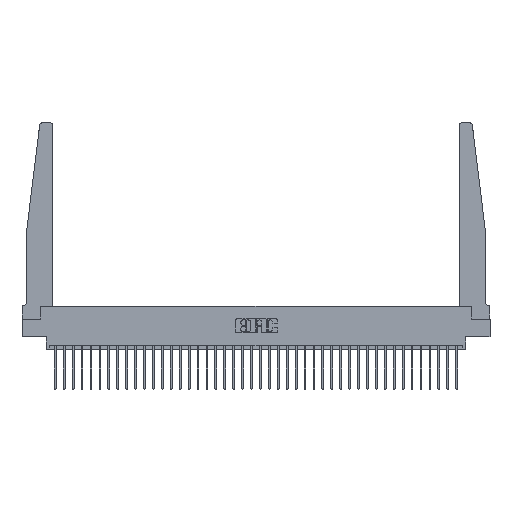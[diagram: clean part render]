
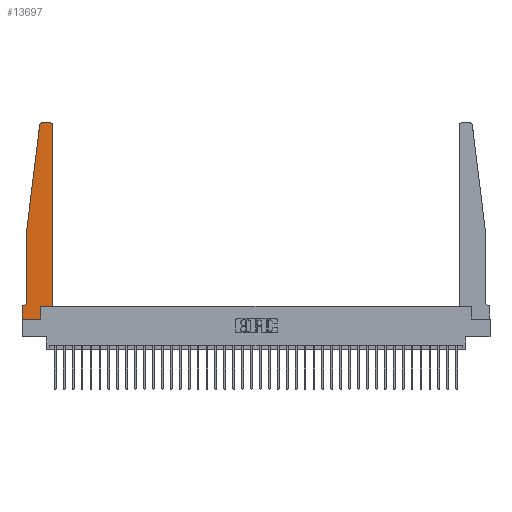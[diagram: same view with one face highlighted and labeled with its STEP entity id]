
A CAD part, top view. The second image highlights one B-rep face of the part: STEP entity #13697.
In plain terms, the highlighted planar face has unit normal (0, 0, 1).
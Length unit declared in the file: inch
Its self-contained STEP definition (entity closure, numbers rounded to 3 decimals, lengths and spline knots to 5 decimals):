
#557 = CARTESIAN_POINT ( 'NONE',  ( 0.24675, 2.72367, 0.37 ) ) ;
#1028 = VECTOR ( 'NONE', #7155, 39.37008 ) ;
#1072 = EDGE_CURVE ( 'NONE', #27527, #33439, #21207, .T. ) ;
#2034 = ORIENTED_EDGE ( 'NONE', *, *, #10402, .T. ) ;
#2082 = CARTESIAN_POINT ( 'NONE',  ( 0., 0., 0.37 ) ) ;
#2559 = LINE ( 'NONE', #28878, #30049 ) ;
#2794 = VERTEX_POINT ( 'NONE', #11726 ) ;
#3166 = ORIENTED_EDGE ( 'NONE', *, *, #26731, .T. ) ;
#4237 = CARTESIAN_POINT ( 'NONE',  ( 0.015, 0.2375, 0.37 ) ) ;
#4277 = DIRECTION ( 'NONE',  ( -0.122, -0.992, 0. ) ) ;
#4312 = VERTEX_POINT ( 'NONE', #4663 ) ;
#4487 = CARTESIAN_POINT ( 'NONE',  ( 0.2605, 0.18, 0.37 ) ) ;
#4598 = DIRECTION ( 'NONE',  ( 1., 0., 0. ) ) ;
#4663 = CARTESIAN_POINT ( 'NONE',  ( 0.395, 2.75, 0.37 ) ) ;
#5028 = EDGE_LOOP ( 'NONE', ( #2034, #30052, #9585, #33416, #3166, #10900, #27820, #19654, #8614, #33044, #7845, #25825 ) ) ;
#5845 = EDGE_CURVE ( 'NONE', #16196, #27527, #28288, .T. ) ;
#6180 = CARTESIAN_POINT ( 'NONE',  ( 0., 0., 0.37 ) ) ;
#6289 = LINE ( 'NONE', #15303, #20442 ) ;
#6762 = EDGE_CURVE ( 'NONE', #14203, #28810, #14049, .T. ) ;
#6897 = DIRECTION ( 'NONE',  ( -1., 0., 0. ) ) ;
#7155 = DIRECTION ( 'NONE',  ( 0., 1., 0. ) ) ;
#7296 = CARTESIAN_POINT ( 'NONE',  ( 0.27653, 2.72, 0.37 ) ) ;
#7845 = ORIENTED_EDGE ( 'NONE', *, *, #17614, .T. ) ;
#8614 = ORIENTED_EDGE ( 'NONE', *, *, #23923, .T. ) ;
#8780 = DIRECTION ( 'NONE',  ( 0., 1., 0. ) ) ;
#8921 = DIRECTION ( 'NONE',  ( 0., -1., 0. ) ) ;
#8934 = LINE ( 'NONE', #4487, #1028 ) ;
#9348 = DIRECTION ( 'NONE',  ( -1., 0., 0. ) ) ;
#9585 = ORIENTED_EDGE ( 'NONE', *, *, #6762, .T. ) ;
#9981 = DIRECTION ( 'NONE',  ( 1., 0., 0. ) ) ;
#10374 = DIRECTION ( 'NONE',  ( -1., 0., 0. ) ) ;
#10402 = EDGE_CURVE ( 'NONE', #4312, #32160, #2559, .T. ) ;
#10419 = CIRCLE ( 'NONE', #15492, 0.05 ) ;
#10900 = ORIENTED_EDGE ( 'NONE', *, *, #31457, .T. ) ;
#11726 = CARTESIAN_POINT ( 'NONE',  ( 0.425, 0.18, 0.37 ) ) ;
#12385 = AXIS2_PLACEMENT_3D ( 'NONE', #14062, #32670, #16736 ) ;
#12436 = VECTOR ( 'NONE', #32806, 39.37008 ) ;
#12508 = CARTESIAN_POINT ( 'NONE',  ( 0.065, 0.2375, 0.37 ) ) ;
#13529 = AXIS2_PLACEMENT_3D ( 'NONE', #7296, #25928, #9981 ) ;
#13697 = ADVANCED_FACE ( 'NONE', ( #20209 ), #19773, .T. ) ;
#14005 = VERTEX_POINT ( 'NONE', #29091 ) ;
#14049 = LINE ( 'NONE', #17521, #34418 ) ;
#14062 = CARTESIAN_POINT ( 'NONE',  ( 0.395, 2.72, 0.37 ) ) ;
#14078 = VECTOR ( 'NONE', #8921, 39.37008 ) ;
#14203 = VERTEX_POINT ( 'NONE', #557 ) ;
#14532 = CARTESIAN_POINT ( 'NONE',  ( 0.425, 2.72, 0.37 ) ) ;
#14556 = CARTESIAN_POINT ( 'NONE',  ( 0., 0.1875, 0.37 ) ) ;
#14597 = CARTESIAN_POINT ( 'NONE',  ( 0.065, 0.1875, 0.37 ) ) ;
#14814 = CARTESIAN_POINT ( 'NONE',  ( 0., 0., 0.37 ) ) ;
#15081 = EDGE_CURVE ( 'NONE', #15214, #4312, #19747, .T. ) ;
#15214 = VERTEX_POINT ( 'NONE', #14532 ) ;
#15303 = CARTESIAN_POINT ( 'NONE',  ( 0.425, 0.18, 0.37 ) ) ;
#15342 = EDGE_CURVE ( 'NONE', #32160, #14203, #18495, .T. ) ;
#15492 = AXIS2_PLACEMENT_3D ( 'NONE', #4237, #22860, #6897 ) ;
#16196 = VERTEX_POINT ( 'NONE', #20981 ) ;
#16736 = DIRECTION ( 'NONE',  ( 1., 0., 0. ) ) ;
#17206 = DIRECTION ( 'NONE',  ( 1., 0., 0. ) ) ;
#17521 = CARTESIAN_POINT ( 'NONE',  ( 0.065, 1.25, 0.37 ) ) ;
#17614 = EDGE_CURVE ( 'NONE', #2794, #15214, #22806, .T. ) ;
#18144 = AXIS2_PLACEMENT_3D ( 'NONE', #14556, #33139, #17206 ) ;
#18495 = CIRCLE ( 'NONE', #13529, 0.03 ) ;
#19383 = CARTESIAN_POINT ( 'NONE',  ( 0.425, 0.18, 0.37 ) ) ;
#19654 = ORIENTED_EDGE ( 'NONE', *, *, #1072, .T. ) ;
#19747 = CIRCLE ( 'NONE', #12385, 0.03 ) ;
#19773 = PLANE ( 'NONE',  #18144 ) ;
#20209 = FACE_OUTER_BOUND ( 'NONE', #5028, .T. ) ;
#20442 = VECTOR ( 'NONE', #4598, 39.37008 ) ;
#20523 = VECTOR ( 'NONE', #9348, 39.37008 ) ;
#20972 = CARTESIAN_POINT ( 'NONE',  ( 0.065, 1.25, 0.37 ) ) ;
#20981 = CARTESIAN_POINT ( 'NONE',  ( 0., 0.1875, 0.37 ) ) ;
#21207 = LINE ( 'NONE', #14814, #27474 ) ;
#21940 = VECTOR ( 'NONE', #8780, 39.37008 ) ;
#22460 = CARTESIAN_POINT ( 'NONE',  ( 0.27653, 2.75, 0.37 ) ) ;
#22806 = LINE ( 'NONE', #19383, #21940 ) ;
#22860 = DIRECTION ( 'NONE',  ( 0., 0., -1. ) ) ;
#23923 = EDGE_CURVE ( 'NONE', #33439, #14005, #8934, .T. ) ;
#24870 = CARTESIAN_POINT ( 'NONE',  ( 0.065, 1.25, 0.37 ) ) ;
#25825 = ORIENTED_EDGE ( 'NONE', *, *, #15081, .T. ) ;
#25900 = EDGE_CURVE ( 'NONE', #14005, #2794, #6289, .T. ) ;
#25928 = DIRECTION ( 'NONE',  ( 0., 0., 1. ) ) ;
#26597 = LINE ( 'NONE', #24870, #14078 ) ;
#26731 = EDGE_CURVE ( 'NONE', #28120, #27822, #10419, .T. ) ;
#27474 = VECTOR ( 'NONE', #28103, 39.37008 ) ;
#27527 = VERTEX_POINT ( 'NONE', #2082 ) ;
#27639 = LINE ( 'NONE', #14597, #20523 ) ;
#27820 = ORIENTED_EDGE ( 'NONE', *, *, #5845, .T. ) ;
#27822 = VERTEX_POINT ( 'NONE', #32755 ) ;
#27844 = EDGE_CURVE ( 'NONE', #28810, #28120, #26597, .T. ) ;
#28103 = DIRECTION ( 'NONE',  ( 1., 0., 0. ) ) ;
#28120 = VERTEX_POINT ( 'NONE', #12508 ) ;
#28288 = LINE ( 'NONE', #6180, #12436 ) ;
#28810 = VERTEX_POINT ( 'NONE', #20972 ) ;
#28878 = CARTESIAN_POINT ( 'NONE',  ( 0.25, 2.75, 0.37 ) ) ;
#29091 = CARTESIAN_POINT ( 'NONE',  ( 0.2605, 0.18, 0.37 ) ) ;
#30049 = VECTOR ( 'NONE', #10374, 39.37008 ) ;
#30052 = ORIENTED_EDGE ( 'NONE', *, *, #15342, .T. ) ;
#30947 = CARTESIAN_POINT ( 'NONE',  ( 0.2605, 0., 0.37 ) ) ;
#31457 = EDGE_CURVE ( 'NONE', #27822, #16196, #27639, .T. ) ;
#32160 = VERTEX_POINT ( 'NONE', #22460 ) ;
#32670 = DIRECTION ( 'NONE',  ( 0., 0., 1. ) ) ;
#32755 = CARTESIAN_POINT ( 'NONE',  ( 0.015, 0.1875, 0.37 ) ) ;
#32806 = DIRECTION ( 'NONE',  ( 0., -1., 0. ) ) ;
#33044 = ORIENTED_EDGE ( 'NONE', *, *, #25900, .T. ) ;
#33139 = DIRECTION ( 'NONE',  ( 0., 0., 1. ) ) ;
#33416 = ORIENTED_EDGE ( 'NONE', *, *, #27844, .T. ) ;
#33439 = VERTEX_POINT ( 'NONE', #30947 ) ;
#34418 = VECTOR ( 'NONE', #4277, 39.37008 ) ;
